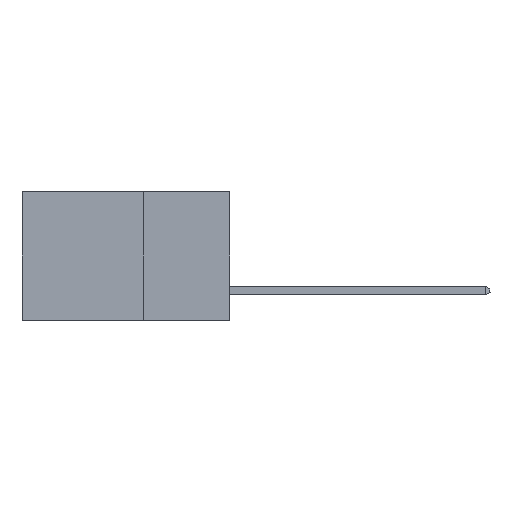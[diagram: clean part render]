
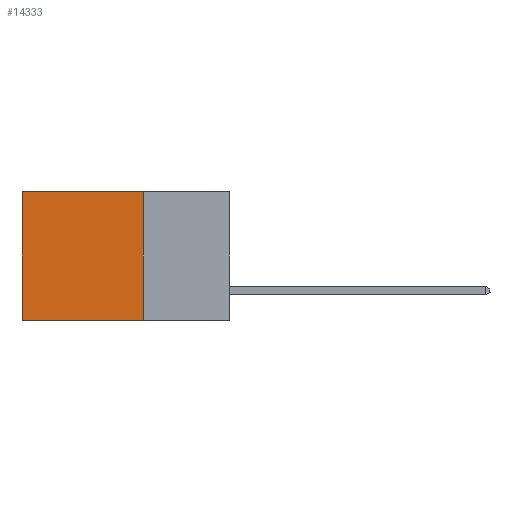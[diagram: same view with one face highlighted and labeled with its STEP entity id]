
A CAD part, left-side view. The second image highlights one B-rep face of the part: STEP entity #14333.
In plain terms, the highlighted planar face has unit normal (-1, 0, 0).
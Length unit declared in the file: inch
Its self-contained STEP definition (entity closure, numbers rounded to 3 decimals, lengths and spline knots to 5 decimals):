
#574 = VECTOR ( 'NONE', #11104, 39.37008 ) ;
#1635 = DIRECTION ( 'NONE',  ( 0., 0., -1. ) ) ;
#3041 = VERTEX_POINT ( 'NONE', #14997 ) ;
#3380 = VECTOR ( 'NONE', #31823, 39.37008 ) ;
#9395 = VERTEX_POINT ( 'NONE', #31573 ) ;
#9652 = PLANE ( 'NONE',  #17668 ) ;
#9728 = DIRECTION ( 'NONE',  ( 0., 0., -1. ) ) ;
#9760 = DIRECTION ( 'NONE',  ( 0., 0., -1. ) ) ;
#10011 = EDGE_CURVE ( 'NONE', #3041, #20466, #23150, .T. ) ;
#11104 = DIRECTION ( 'NONE',  ( 0., 1., 0. ) ) ;
#11468 = CARTESIAN_POINT ( 'NONE',  ( 0.298, 0.25, -0.37 ) ) ;
#11568 = CARTESIAN_POINT ( 'NONE',  ( 0.298, 0.25, -0.37 ) ) ;
#14333 = ADVANCED_FACE ( 'NONE', ( #27009 ), #9652, .F. ) ;
#14395 = VERTEX_POINT ( 'NONE', #23452 ) ;
#14997 = CARTESIAN_POINT ( 'NONE',  ( 0.298, 0.25, 0. ) ) ;
#16000 = EDGE_CURVE ( 'NONE', #20466, #9395, #24536, .T. ) ;
#17015 = LINE ( 'NONE', #26118, #574 ) ;
#17668 = AXIS2_PLACEMENT_3D ( 'NONE', #20388, #19734, #9760 ) ;
#18453 = VECTOR ( 'NONE', #1635, 39.37008 ) ;
#19734 = DIRECTION ( 'NONE',  ( 1., 0., 0. ) ) ;
#20388 = CARTESIAN_POINT ( 'NONE',  ( 0.298, 0.25, 0. ) ) ;
#20466 = VERTEX_POINT ( 'NONE', #11468 ) ;
#20557 = ORIENTED_EDGE ( 'NONE', *, *, #10011, .F. ) ;
#21729 = CARTESIAN_POINT ( 'NONE',  ( 0.298, 0.25, 0. ) ) ;
#23150 = LINE ( 'NONE', #21729, #18453 ) ;
#23434 = EDGE_CURVE ( 'NONE', #3041, #14395, #17015, .T. ) ;
#23452 = CARTESIAN_POINT ( 'NONE',  ( 0.298, 0.6, 0. ) ) ;
#23781 = ORIENTED_EDGE ( 'NONE', *, *, #23434, .T. ) ;
#24536 = LINE ( 'NONE', #11568, #3380 ) ;
#25621 = VECTOR ( 'NONE', #9728, 39.37008 ) ;
#26008 = EDGE_LOOP ( 'NONE', ( #32370, #30281, #20557, #23781 ) ) ;
#26118 = CARTESIAN_POINT ( 'NONE',  ( 0.298, 0.25, 0. ) ) ;
#27009 = FACE_OUTER_BOUND ( 'NONE', #26008, .T. ) ;
#30281 = ORIENTED_EDGE ( 'NONE', *, *, #16000, .F. ) ;
#30983 = EDGE_CURVE ( 'NONE', #14395, #9395, #31467, .T. ) ;
#31467 = LINE ( 'NONE', #32065, #25621 ) ;
#31573 = CARTESIAN_POINT ( 'NONE',  ( 0.298, 0.6, -0.37 ) ) ;
#31823 = DIRECTION ( 'NONE',  ( 0., 1., 0. ) ) ;
#32065 = CARTESIAN_POINT ( 'NONE',  ( 0.298, 0.6, 0. ) ) ;
#32370 = ORIENTED_EDGE ( 'NONE', *, *, #30983, .T. ) ;
